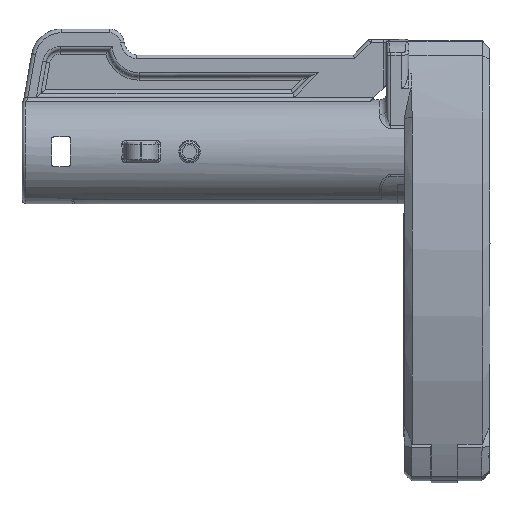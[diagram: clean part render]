
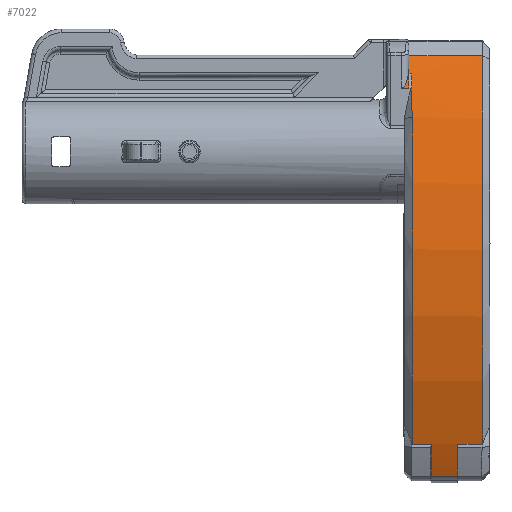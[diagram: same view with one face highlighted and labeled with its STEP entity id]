
A CAD part, top view. The second image highlights one B-rep face of the part: STEP entity #7022.
In plain terms, the highlighted cylindrical face has radius 180.483 mm (diameter 360.965 mm), a partial arc.
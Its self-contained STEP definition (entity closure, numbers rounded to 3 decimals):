
#95=(
BOUNDED_CURVE()
B_SPLINE_CURVE(2,(#10905,#10906,#10907),.UNSPECIFIED.,.F.,.F.)
B_SPLINE_CURVE_WITH_KNOTS((3,3),(0.503,0.753),
 .UNSPECIFIED.)
CURVE()
GEOMETRIC_REPRESENTATION_ITEM()
RATIONAL_B_SPLINE_CURVE((1.,1.,1.))
REPRESENTATION_ITEM('')
);
#102=ELLIPSE('',#7459,180.486,180.483);
#104=ELLIPSE('',#7462,180.486,180.483);
#105=ELLIPSE('',#7468,180.486,180.483);
#188=CYLINDRICAL_SURFACE('',#7463,180.483);
#321=CIRCLE('',#7464,180.483);
#322=CIRCLE('',#7465,180.483);
#323=CIRCLE('',#7466,180.483);
#324=CIRCLE('',#7467,180.483);
#670=B_SPLINE_CURVE_WITH_KNOTS('',3,(#10831,#10832,#10833,#10834,#10835,
#10836),.UNSPECIFIED.,.F.,.F.,(4,2,4),(0.,0.05,0.1),
 .UNSPECIFIED.);
#672=B_SPLINE_CURVE_WITH_KNOTS('',3,(#10862,#10863,#10864,#10865,#10866,
#10867,#10868),.UNSPECIFIED.,.F.,.F.,(4,3,4),(-0.033,-0.028,
-0.023),.UNSPECIFIED.);
#673=B_SPLINE_CURVE_WITH_KNOTS('',3,(#10888,#10889,#10890,#10891,#10892,
#10893,#10894,#10895,#10896,#10897,#10898,#10899,#10900,#10901,#10902,#10903,
#10904),.UNSPECIFIED.,.F.,.F.,(4,2,2,2,2,2,3,4),(2.378,2.698,
2.86,3.023,3.155,3.186,3.218,
3.219),.UNSPECIFIED.);
#960=FACE_OUTER_BOUND('',#1389,.T.);
#1389=EDGE_LOOP('',(#5041,#5042,#5043,#5044,#5045,#5046,#5047,#5048,#5049,
#5050,#5051,#5052,#5053,#5054,#5055,#5056));
#1948=LINE('',#10860,#2477);
#1949=LINE('',#10872,#2478);
#1950=LINE('',#10876,#2479);
#1951=LINE('',#10880,#2480);
#1952=LINE('',#10884,#2481);
#2477=VECTOR('',#8509,10.);
#2478=VECTOR('',#8512,1000.);
#2479=VECTOR('',#8515,1000.);
#2480=VECTOR('',#8518,1000.);
#2481=VECTOR('',#8521,1000.);
#2963=VERTEX_POINT('',#10829);
#2964=VERTEX_POINT('',#10830);
#2966=VERTEX_POINT('',#10849);
#2968=VERTEX_POINT('',#10855);
#2969=VERTEX_POINT('',#10859);
#2970=VERTEX_POINT('',#10861);
#2971=VERTEX_POINT('',#10869);
#2972=VERTEX_POINT('',#10871);
#2973=VERTEX_POINT('',#10873);
#2974=VERTEX_POINT('',#10875);
#2975=VERTEX_POINT('',#10877);
#2976=VERTEX_POINT('',#10879);
#2977=VERTEX_POINT('',#10881);
#2978=VERTEX_POINT('',#10883);
#2979=VERTEX_POINT('',#10885);
#2980=VERTEX_POINT('',#10887);
#3727=EDGE_CURVE('',#2963,#2964,#670,.T.);
#3730=EDGE_CURVE('',#2966,#2963,#102,.T.);
#3733=EDGE_CURVE('',#2964,#2968,#104,.T.);
#3735=EDGE_CURVE('',#2968,#2969,#1948,.T.);
#3736=EDGE_CURVE('',#2970,#2969,#672,.T.);
#3737=EDGE_CURVE('',#2971,#2970,#321,.T.);
#3738=EDGE_CURVE('',#2972,#2971,#1949,.T.);
#3739=EDGE_CURVE('',#2973,#2972,#322,.T.);
#3740=EDGE_CURVE('',#2973,#2974,#1950,.T.);
#3741=EDGE_CURVE('',#2975,#2974,#323,.T.);
#3742=EDGE_CURVE('',#2976,#2975,#1951,.T.);
#3743=EDGE_CURVE('',#2977,#2976,#324,.T.);
#3744=EDGE_CURVE('',#2977,#2978,#1952,.F.);
#3745=EDGE_CURVE('',#2978,#2979,#105,.T.);
#3746=EDGE_CURVE('',#2980,#2979,#673,.F.);
#3747=EDGE_CURVE('',#2980,#2966,#95,.T.);
#5041=ORIENTED_EDGE('',*,*,#3727,.T.);
#5042=ORIENTED_EDGE('',*,*,#3733,.T.);
#5043=ORIENTED_EDGE('',*,*,#3735,.T.);
#5044=ORIENTED_EDGE('',*,*,#3736,.F.);
#5045=ORIENTED_EDGE('',*,*,#3737,.F.);
#5046=ORIENTED_EDGE('',*,*,#3738,.F.);
#5047=ORIENTED_EDGE('',*,*,#3739,.F.);
#5048=ORIENTED_EDGE('',*,*,#3740,.T.);
#5049=ORIENTED_EDGE('',*,*,#3741,.F.);
#5050=ORIENTED_EDGE('',*,*,#3742,.F.);
#5051=ORIENTED_EDGE('',*,*,#3743,.F.);
#5052=ORIENTED_EDGE('',*,*,#3744,.T.);
#5053=ORIENTED_EDGE('',*,*,#3745,.T.);
#5054=ORIENTED_EDGE('',*,*,#3746,.F.);
#5055=ORIENTED_EDGE('',*,*,#3747,.T.);
#5056=ORIENTED_EDGE('',*,*,#3730,.T.);
#7022=ADVANCED_FACE('',(#960),#188,.T.);
#7459=AXIS2_PLACEMENT_3D('',#10850,#8497,#8498);
#7462=AXIS2_PLACEMENT_3D('',#10856,#8504,#8505);
#7463=AXIS2_PLACEMENT_3D('',#10858,#8507,#8508);
#7464=AXIS2_PLACEMENT_3D('',#10870,#8510,#8511);
#7465=AXIS2_PLACEMENT_3D('',#10874,#8513,#8514);
#7466=AXIS2_PLACEMENT_3D('',#10878,#8516,#8517);
#7467=AXIS2_PLACEMENT_3D('',#10882,#8519,#8520);
#7468=AXIS2_PLACEMENT_3D('',#10886,#8522,#8523);
#8497=DIRECTION('center_axis',(0.006,1.,0.));
#8498=DIRECTION('ref_axis',(-0.999,0.006,-0.053));
#8504=DIRECTION('center_axis',(-0.006,-1.,0.));
#8505=DIRECTION('ref_axis',(-0.999,0.006,-0.053));
#8507=DIRECTION('center_axis',(0.,-1.,
0.));
#8508=DIRECTION('ref_axis',(-0.954,0.,0.301));
#8509=DIRECTION('',(0.006,1.,0.019));
#8510=DIRECTION('center_axis',(0.,1.,0.));
#8511=DIRECTION('ref_axis',(-0.999,0.,-0.051));
#8512=DIRECTION('',(0.,1.,0.));
#8513=DIRECTION('center_axis',(0.,1.,0.));
#8514=DIRECTION('ref_axis',(-0.954,0.,0.301));
#8515=DIRECTION('',(0.,-1.,0.));
#8516=DIRECTION('center_axis',(0.,-1.,
0.));
#8517=DIRECTION('ref_axis',(-0.954,0.,0.301));
#8518=DIRECTION('',(0.,1.,0.));
#8519=DIRECTION('center_axis',(0.,-1.,
0.));
#8520=DIRECTION('ref_axis',(-1.,0.,-0.009));
#8521=DIRECTION('',(0.,-1.,0.));
#8522=DIRECTION('center_axis',(-0.006,-1.,
0.));
#8523=DIRECTION('ref_axis',(-0.999,0.006,-0.053));
#10829=CARTESIAN_POINT('',(16.14,28.9,92.007));
#10830=CARTESIAN_POINT('',(16.124,27.9,91.959));
#10831=CARTESIAN_POINT('Ctrl Pts',(16.14,28.9,92.007));
#10832=CARTESIAN_POINT('Ctrl Pts',(16.138,28.733,91.999));
#10833=CARTESIAN_POINT('Ctrl Pts',(16.135,28.567,91.991));
#10834=CARTESIAN_POINT('Ctrl Pts',(16.129,28.233,91.975));
#10835=CARTESIAN_POINT('Ctrl Pts',(16.127,28.067,91.967));
#10836=CARTESIAN_POINT('Ctrl Pts',(16.124,27.9,91.959));
#10849=CARTESIAN_POINT('',(14.558,28.91,87.06));
#10850=CARTESIAN_POINT('Origin',(187.235,27.947,34.558));
#10855=CARTESIAN_POINT('',(14.552,27.911,87.041));
#10856=CARTESIAN_POINT('Origin',(187.235,26.947,34.558));
#10858=CARTESIAN_POINT('Origin',(187.235,3.271,34.558));
#10859=CARTESIAN_POINT('',(14.554,28.195,87.047));
#10860=CARTESIAN_POINT('',(14.555,28.411,87.051));
#10861=CARTESIAN_POINT('',(11.903,27.772,77.365));
#10862=CARTESIAN_POINT('Ctrl Pts',(11.903,27.772,77.365));
#10863=CARTESIAN_POINT('Ctrl Pts',(12.313,27.772,79.046));
#10864=CARTESIAN_POINT('Ctrl Pts',(12.748,27.801,80.723));
#10865=CARTESIAN_POINT('Ctrl Pts',(13.207,27.872,82.392));
#10866=CARTESIAN_POINT('Ctrl Pts',(13.636,27.939,83.952));
#10867=CARTESIAN_POINT('Ctrl Pts',(14.085,28.042,85.505));
#10868=CARTESIAN_POINT('Ctrl Pts',(14.554,28.195,87.047));
#10869=CARTESIAN_POINT('',(20.411,27.771,-34.317));
#10870=CARTESIAN_POINT('Origin',(187.235,27.771,34.558));
#10871=CARTESIAN_POINT('',(20.411,21.271,-34.317));
#10872=CARTESIAN_POINT('',(20.411,30.271,-34.317));
#10873=CARTESIAN_POINT('',(25.397,21.271,-45.332));
#10874=CARTESIAN_POINT('Origin',(187.235,21.271,34.558));
#10875=CARTESIAN_POINT('',(25.397,12.271,-45.332));
#10876=CARTESIAN_POINT('',(25.397,12.271,-45.332));
#10877=CARTESIAN_POINT('',(20.411,12.271,-34.317));
#10878=CARTESIAN_POINT('Origin',(187.235,12.271,34.558));
#10879=CARTESIAN_POINT('',(20.411,3.771,-34.317));
#10880=CARTESIAN_POINT('',(20.411,30.271,-34.317));
#10881=CARTESIAN_POINT('',(18.346,3.772,98.2));
#10882=CARTESIAN_POINT('Origin',(187.235,3.771,34.558));
#10883=CARTESIAN_POINT('',(18.346,28.886,98.2));
#10884=CARTESIAN_POINT('',(18.346,136.115,98.199));
#10885=CARTESIAN_POINT('',(17.096,28.894,94.778));
#10886=CARTESIAN_POINT('Origin',(187.235,27.947,34.558));
#10887=CARTESIAN_POINT('',(14.572,31.41,87.107));
#10888=CARTESIAN_POINT('Ctrl Pts',(17.096,28.894,94.778));
#10889=CARTESIAN_POINT('Ctrl Pts',(16.739,28.896,93.769));
#10890=CARTESIAN_POINT('Ctrl Pts',(16.358,28.974,92.664));
#10891=CARTESIAN_POINT('Ctrl Pts',(15.812,29.238,91.024));
#10892=CARTESIAN_POINT('Ctrl Pts',(15.633,29.351,90.478));
#10893=CARTESIAN_POINT('Ctrl Pts',(15.293,29.637,89.423));
#10894=CARTESIAN_POINT('Ctrl Pts',(15.132,29.808,88.914));
#10895=CARTESIAN_POINT('Ctrl Pts',(14.864,30.212,88.059));
#10896=CARTESIAN_POINT('Ctrl Pts',(14.727,30.469,87.615));
#10897=CARTESIAN_POINT('Ctrl Pts',(14.624,30.886,87.278));
#10898=CARTESIAN_POINT('Ctrl Pts',(14.606,30.98,87.217));
#10899=CARTESIAN_POINT('Ctrl Pts',(14.579,31.183,87.131));
#10900=CARTESIAN_POINT('Ctrl Pts',(14.572,31.292,87.107));
#10901=CARTESIAN_POINT('Ctrl Pts',(14.572,31.396,87.107));
#10902=CARTESIAN_POINT('Ctrl Pts',(14.572,31.401,87.107));
#10903=CARTESIAN_POINT('Ctrl Pts',(14.572,31.406,87.107));
#10904=CARTESIAN_POINT('Ctrl Pts',(14.572,31.41,87.107));
#10905=CARTESIAN_POINT('Ctrl Pts',(14.572,31.41,87.107));
#10906=CARTESIAN_POINT('Ctrl Pts',(14.565,30.16,87.084));
#10907=CARTESIAN_POINT('Ctrl Pts',(14.558,28.91,87.06));
